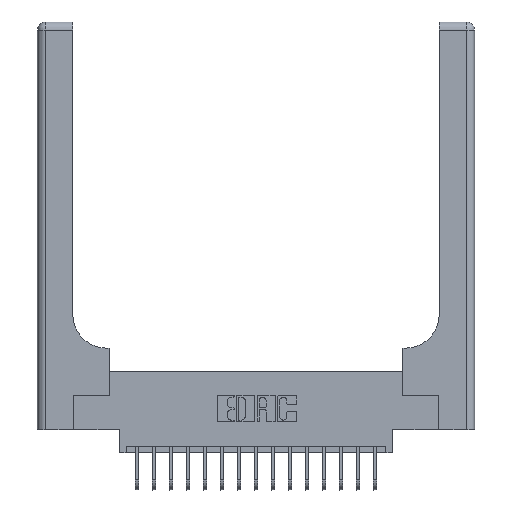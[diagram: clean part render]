
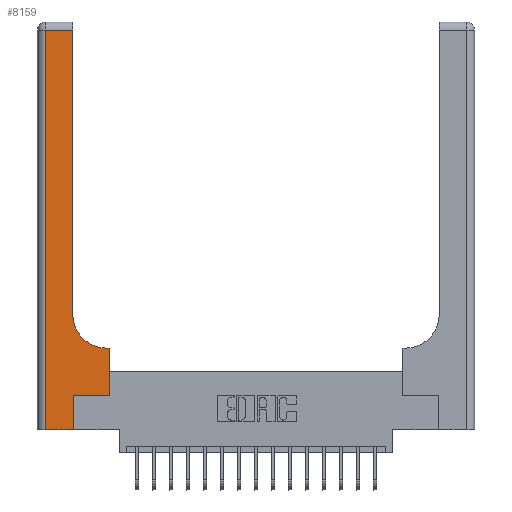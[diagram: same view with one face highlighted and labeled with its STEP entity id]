
A CAD part, top view. The second image highlights one B-rep face of the part: STEP entity #8159.
In plain terms, the highlighted planar face has unit normal (0, 0, 1).
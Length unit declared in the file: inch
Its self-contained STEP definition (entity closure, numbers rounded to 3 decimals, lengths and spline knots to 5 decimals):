
#96 = EDGE_CURVE ( 'NONE', #9962, #4403, #15397, .T. ) ;
#160 = CARTESIAN_POINT ( 'NONE',  ( 0.51, 0.6, 0.37 ) ) ;
#325 = ORIENTED_EDGE ( 'NONE', *, *, #16162, .T. ) ;
#424 = ORIENTED_EDGE ( 'NONE', *, *, #18015, .T. ) ;
#875 = LINE ( 'NONE', #8407, #17425 ) ;
#1185 = VECTOR ( 'NONE', #14406, 39.37008 ) ;
#1299 = LINE ( 'NONE', #11478, #1185 ) ;
#2002 = CARTESIAN_POINT ( 'NONE',  ( 0.51, 0.85, 0.37 ) ) ;
#2176 = DIRECTION ( 'NONE',  ( 0., 0., -1. ) ) ;
#2466 = LINE ( 'NONE', #13969, #12258 ) ;
#2486 = ORIENTED_EDGE ( 'NONE', *, *, #7099, .T. ) ;
#2662 = CARTESIAN_POINT ( 'NONE',  ( 0.06, 3., 0.37 ) ) ;
#2890 = VECTOR ( 'NONE', #14528, 39.37008 ) ;
#2955 = AXIS2_PLACEMENT_3D ( 'NONE', #16094, #4610, #13335 ) ;
#3012 = EDGE_CURVE ( 'NONE', #7901, #13852, #2466, .T. ) ;
#3049 = CARTESIAN_POINT ( 'NONE',  ( 0.265, 0., 0.37 ) ) ;
#3469 = LINE ( 'NONE', #7573, #14721 ) ;
#4000 = CARTESIAN_POINT ( 'NONE',  ( 0.528, 0.6, 0.37 ) ) ;
#4283 = CARTESIAN_POINT ( 'NONE',  ( 0.26, 0.85, 0.37 ) ) ;
#4403 = VERTEX_POINT ( 'NONE', #4283 ) ;
#4462 = VERTEX_POINT ( 'NONE', #3049 ) ;
#4595 = ORIENTED_EDGE ( 'NONE', *, *, #10123, .T. ) ;
#4610 = DIRECTION ( 'NONE',  ( 0., 0., -1. ) ) ;
#5263 = EDGE_CURVE ( 'NONE', #13860, #4462, #1299, .T. ) ;
#5531 = DIRECTION ( 'NONE',  ( 0., -1., 0. ) ) ;
#5951 = PLANE ( 'NONE',  #2955 ) ;
#6573 = CARTESIAN_POINT ( 'NONE',  ( 0.528, 0.25, 0.37 ) ) ;
#6862 = CARTESIAN_POINT ( 'NONE',  ( 0.06, 0., 0.37 ) ) ;
#7099 = EDGE_CURVE ( 'NONE', #13852, #13860, #17022, .T. ) ;
#7257 = VERTEX_POINT ( 'NONE', #6573 ) ;
#7573 = CARTESIAN_POINT ( 'NONE',  ( 0.528, 0.25, 0.37 ) ) ;
#7690 = ORIENTED_EDGE ( 'NONE', *, *, #96, .T. ) ;
#7901 = VERTEX_POINT ( 'NONE', #10117 ) ;
#8047 = CARTESIAN_POINT ( 'NONE',  ( 0.26, 0.6, 0.37 ) ) ;
#8159 = ADVANCED_FACE ( 'NONE', ( #11733 ), #5951, .F. ) ;
#8393 = EDGE_LOOP ( 'NONE', ( #325, #11411, #2486, #13328, #4595, #424, #15080, #16243, #7690 ) ) ;
#8407 = CARTESIAN_POINT ( 'NONE',  ( 0.26, 3., 0.37 ) ) ;
#8448 = VERTEX_POINT ( 'NONE', #4000 ) ;
#8815 = CARTESIAN_POINT ( 'NONE',  ( 0.265, 0.25, 0.37 ) ) ;
#9279 = DIRECTION ( 'NONE',  ( 0., 1., 0. ) ) ;
#9332 = DIRECTION ( 'NONE',  ( 1., 0., 0. ) ) ;
#9834 = DIRECTION ( 'NONE',  ( -1., 0., 0. ) ) ;
#9962 = VERTEX_POINT ( 'NONE', #160 ) ;
#9988 = EDGE_CURVE ( 'NONE', #7257, #8448, #3469, .T. ) ;
#10117 = CARTESIAN_POINT ( 'NONE',  ( 0.26, 2.94, 0.37 ) ) ;
#10123 = EDGE_CURVE ( 'NONE', #4462, #18422, #12588, .T. ) ;
#10166 = LINE ( 'NONE', #11869, #2890 ) ;
#11069 = CARTESIAN_POINT ( 'NONE',  ( 0.265, 0., 0.37 ) ) ;
#11329 = VECTOR ( 'NONE', #9834, 39.37008 ) ;
#11355 = VECTOR ( 'NONE', #5531, 39.37008 ) ;
#11411 = ORIENTED_EDGE ( 'NONE', *, *, #3012, .T. ) ;
#11478 = CARTESIAN_POINT ( 'NONE',  ( 0., 0., 0.37 ) ) ;
#11733 = FACE_OUTER_BOUND ( 'NONE', #8393, .T. ) ;
#11869 = CARTESIAN_POINT ( 'NONE',  ( 0.265, 0.25, 0.37 ) ) ;
#12258 = VECTOR ( 'NONE', #15481, 39.37008 ) ;
#12293 = DIRECTION ( 'NONE',  ( 0., 1., 0. ) ) ;
#12547 = VECTOR ( 'NONE', #16860, 39.37008 ) ;
#12588 = LINE ( 'NONE', #11069, #12547 ) ;
#13328 = ORIENTED_EDGE ( 'NONE', *, *, #5263, .T. ) ;
#13335 = DIRECTION ( 'NONE',  ( -1., 0., 0. ) ) ;
#13852 = VERTEX_POINT ( 'NONE', #15664 ) ;
#13860 = VERTEX_POINT ( 'NONE', #6862 ) ;
#13969 = CARTESIAN_POINT ( 'NONE',  ( 0., 2.94, 0.37 ) ) ;
#14406 = DIRECTION ( 'NONE',  ( 1., 0., 0. ) ) ;
#14528 = DIRECTION ( 'NONE',  ( 1., 0., 0. ) ) ;
#14700 = EDGE_CURVE ( 'NONE', #8448, #9962, #17060, .T. ) ;
#14721 = VECTOR ( 'NONE', #9279, 39.37008 ) ;
#15080 = ORIENTED_EDGE ( 'NONE', *, *, #9988, .T. ) ;
#15397 = CIRCLE ( 'NONE', #16974, 0.25 ) ;
#15481 = DIRECTION ( 'NONE',  ( -1., 0., 0. ) ) ;
#15664 = CARTESIAN_POINT ( 'NONE',  ( 0.06, 2.94, 0.37 ) ) ;
#16094 = CARTESIAN_POINT ( 'NONE',  ( 0., 3., 0.37 ) ) ;
#16162 = EDGE_CURVE ( 'NONE', #4403, #7901, #875, .T. ) ;
#16243 = ORIENTED_EDGE ( 'NONE', *, *, #14700, .T. ) ;
#16860 = DIRECTION ( 'NONE',  ( 0., 1., 0. ) ) ;
#16974 = AXIS2_PLACEMENT_3D ( 'NONE', #2002, #2176, #9332 ) ;
#17022 = LINE ( 'NONE', #2662, #11355 ) ;
#17060 = LINE ( 'NONE', #8047, #11329 ) ;
#17425 = VECTOR ( 'NONE', #12293, 39.37008 ) ;
#18015 = EDGE_CURVE ( 'NONE', #18422, #7257, #10166, .T. ) ;
#18422 = VERTEX_POINT ( 'NONE', #8815 ) ;
